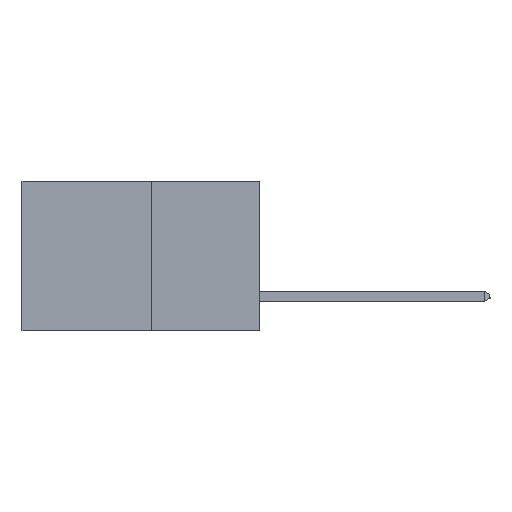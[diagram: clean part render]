
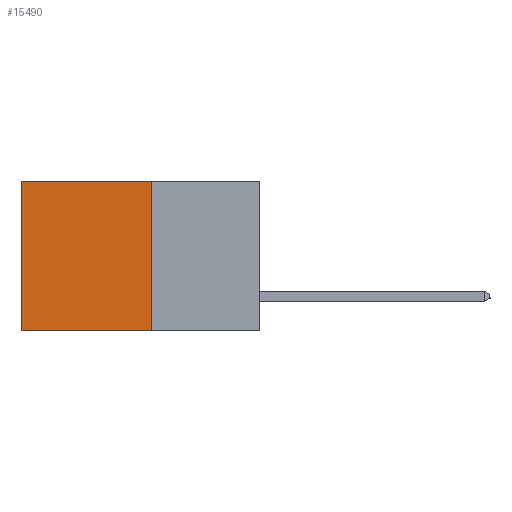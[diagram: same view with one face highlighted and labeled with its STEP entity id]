
A CAD part, left-side view. The second image highlights one B-rep face of the part: STEP entity #15490.
In plain terms, the highlighted planar face has unit normal (-1, 0, 0).
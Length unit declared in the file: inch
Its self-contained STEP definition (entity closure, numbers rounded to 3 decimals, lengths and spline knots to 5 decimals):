
#61 = VECTOR ( 'NONE', #8140, 39.37008 ) ;
#369 = CARTESIAN_POINT ( 'NONE',  ( 0.277, 0.59, 0. ) ) ;
#407 = VERTEX_POINT ( 'NONE', #369 ) ;
#1543 = ORIENTED_EDGE ( 'NONE', *, *, #12916, .T. ) ;
#1736 = CARTESIAN_POINT ( 'NONE',  ( 0.277, 0.27, 0. ) ) ;
#2347 = LINE ( 'NONE', #9274, #15517 ) ;
#2349 = ORIENTED_EDGE ( 'NONE', *, *, #13227, .T. ) ;
#3478 = FACE_OUTER_BOUND ( 'NONE', #7609, .T. ) ;
#3574 = ORIENTED_EDGE ( 'NONE', *, *, #15079, .F. ) ;
#5502 = VERTEX_POINT ( 'NONE', #6887 ) ;
#5615 = CARTESIAN_POINT ( 'NONE',  ( 0.277, 0.27, 0. ) ) ;
#6335 = VECTOR ( 'NONE', #14154, 39.37008 ) ;
#6820 = AXIS2_PLACEMENT_3D ( 'NONE', #12597, #14916, #7750 ) ;
#6874 = CARTESIAN_POINT ( 'NONE',  ( 0.277, 0.59, -0.37 ) ) ;
#6887 = CARTESIAN_POINT ( 'NONE',  ( 0.277, 0.59, -0.37 ) ) ;
#7536 = VERTEX_POINT ( 'NONE', #10996 ) ;
#7609 = EDGE_LOOP ( 'NONE', ( #2349, #3574, #13020, #1543 ) ) ;
#7750 = DIRECTION ( 'NONE',  ( 0., 0., -1. ) ) ;
#8140 = DIRECTION ( 'NONE',  ( 0., 0., -1. ) ) ;
#8195 = CARTESIAN_POINT ( 'NONE',  ( 0.277, 0.27, -0.37 ) ) ;
#8351 = VECTOR ( 'NONE', #9276, 39.37008 ) ;
#9274 = CARTESIAN_POINT ( 'NONE',  ( 0.277, 0.27, -0.37 ) ) ;
#9276 = DIRECTION ( 'NONE',  ( 0., 1., 0. ) ) ;
#9881 = LINE ( 'NONE', #6874, #61 ) ;
#10996 = CARTESIAN_POINT ( 'NONE',  ( 0.277, 0.27, -0.37 ) ) ;
#11038 = EDGE_CURVE ( 'NONE', #12297, #7536, #2347, .T. ) ;
#12297 = VERTEX_POINT ( 'NONE', #1736 ) ;
#12597 = CARTESIAN_POINT ( 'NONE',  ( 0.277, 0.27, -0.37 ) ) ;
#12812 = LINE ( 'NONE', #8195, #6335 ) ;
#12916 = EDGE_CURVE ( 'NONE', #12297, #407, #14327, .T. ) ;
#13020 = ORIENTED_EDGE ( 'NONE', *, *, #11038, .F. ) ;
#13227 = EDGE_CURVE ( 'NONE', #407, #5502, #9881, .T. ) ;
#13701 = PLANE ( 'NONE',  #6820 ) ;
#14056 = DIRECTION ( 'NONE',  ( 0., 0., -1. ) ) ;
#14154 = DIRECTION ( 'NONE',  ( 0., 1., 0. ) ) ;
#14327 = LINE ( 'NONE', #5615, #8351 ) ;
#14916 = DIRECTION ( 'NONE',  ( 1., 0., 0. ) ) ;
#15079 = EDGE_CURVE ( 'NONE', #7536, #5502, #12812, .T. ) ;
#15490 = ADVANCED_FACE ( 'NONE', ( #3478 ), #13701, .F. ) ;
#15517 = VECTOR ( 'NONE', #14056, 39.37008 ) ;
